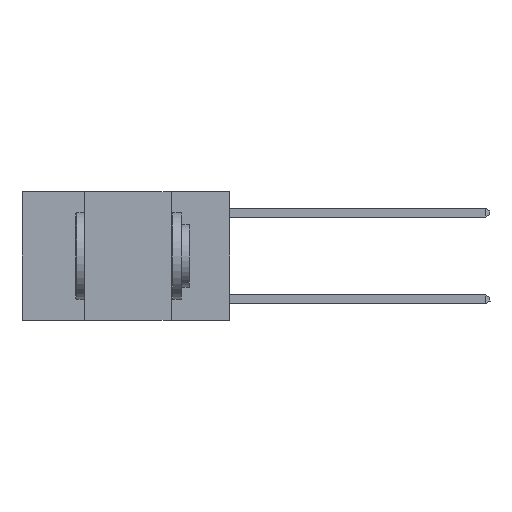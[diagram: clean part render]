
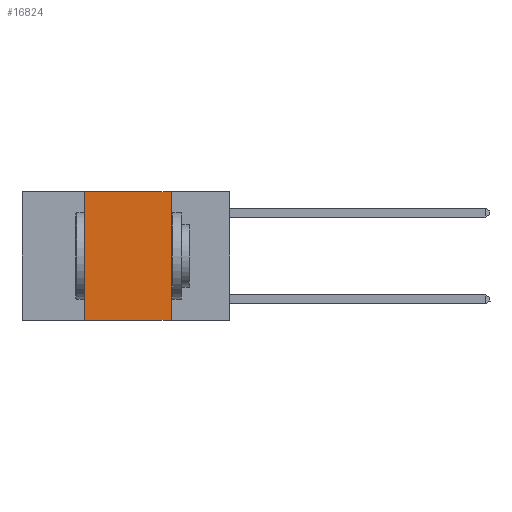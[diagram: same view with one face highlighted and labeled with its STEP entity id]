
A CAD part, left-side view. The second image highlights one B-rep face of the part: STEP entity #16824.
In plain terms, the highlighted planar face has unit normal (-1, 0, 0).
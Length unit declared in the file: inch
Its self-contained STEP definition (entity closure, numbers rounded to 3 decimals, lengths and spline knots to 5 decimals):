
#249 = CARTESIAN_POINT ( 'NONE',  ( 0., 0.42, -0.37 ) ) ;
#396 = ORIENTED_EDGE ( 'NONE', *, *, #6928, .F. ) ;
#653 = CARTESIAN_POINT ( 'NONE',  ( 0., 0.17, 0. ) ) ;
#713 = LINE ( 'NONE', #13073, #4413 ) ;
#1430 = DIRECTION ( 'NONE',  ( 0., 0., -1. ) ) ;
#2778 = VERTEX_POINT ( 'NONE', #653 ) ;
#2998 = CARTESIAN_POINT ( 'NONE',  ( 0., 0.6, -0.37 ) ) ;
#4413 = VECTOR ( 'NONE', #11790, 39.37008 ) ;
#4426 = VECTOR ( 'NONE', #8449, 39.37008 ) ;
#4500 = VECTOR ( 'NONE', #12690, 39.37008 ) ;
#4703 = LINE ( 'NONE', #14206, #11990 ) ;
#5601 = CARTESIAN_POINT ( 'NONE',  ( 0., 0.6, 0. ) ) ;
#6174 = ORIENTED_EDGE ( 'NONE', *, *, #16512, .F. ) ;
#6219 = EDGE_CURVE ( 'NONE', #16552, #14594, #7349, .T. ) ;
#6671 = ORIENTED_EDGE ( 'NONE', *, *, #6219, .T. ) ;
#6928 = EDGE_CURVE ( 'NONE', #17605, #2778, #12782, .T. ) ;
#7349 = LINE ( 'NONE', #2998, #4426 ) ;
#8363 = DIRECTION ( 'NONE',  ( 1., 0., 0. ) ) ;
#8449 = DIRECTION ( 'NONE',  ( 0., -1., 0. ) ) ;
#8785 = EDGE_LOOP ( 'NONE', ( #6174, #396, #16485, #6671 ) ) ;
#11520 = EDGE_CURVE ( 'NONE', #16552, #17605, #713, .T. ) ;
#11790 = DIRECTION ( 'NONE',  ( 0., 0., 1. ) ) ;
#11990 = VECTOR ( 'NONE', #17201, 39.37008 ) ;
#12690 = DIRECTION ( 'NONE',  ( 0., -1., 0. ) ) ;
#12782 = LINE ( 'NONE', #5601, #4500 ) ;
#13073 = CARTESIAN_POINT ( 'NONE',  ( 0., 0.42, 0. ) ) ;
#13706 = CARTESIAN_POINT ( 'NONE',  ( 0., 0.6, 0. ) ) ;
#14085 = PLANE ( 'NONE',  #17368 ) ;
#14206 = CARTESIAN_POINT ( 'NONE',  ( 0., 0.17, 0. ) ) ;
#14594 = VERTEX_POINT ( 'NONE', #14804 ) ;
#14804 = CARTESIAN_POINT ( 'NONE',  ( 0., 0.17, -0.37 ) ) ;
#14817 = CARTESIAN_POINT ( 'NONE',  ( 0., 0.42, 0. ) ) ;
#16485 = ORIENTED_EDGE ( 'NONE', *, *, #11520, .F. ) ;
#16512 = EDGE_CURVE ( 'NONE', #2778, #14594, #4703, .T. ) ;
#16552 = VERTEX_POINT ( 'NONE', #249 ) ;
#16824 = ADVANCED_FACE ( 'NONE', ( #18095 ), #14085, .F. ) ;
#17201 = DIRECTION ( 'NONE',  ( 0., 0., -1. ) ) ;
#17368 = AXIS2_PLACEMENT_3D ( 'NONE', #13706, #8363, #1430 ) ;
#17605 = VERTEX_POINT ( 'NONE', #14817 ) ;
#18095 = FACE_OUTER_BOUND ( 'NONE', #8785, .T. ) ;
